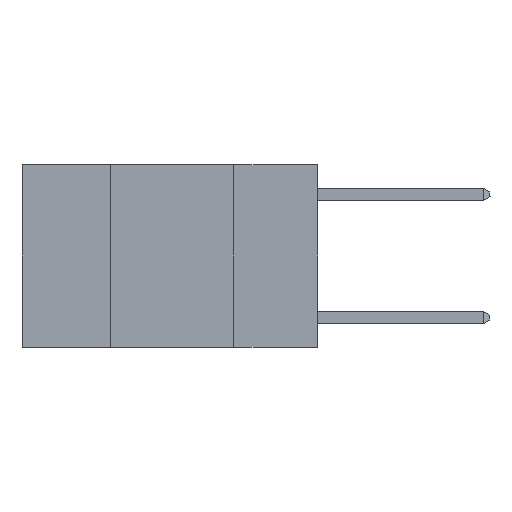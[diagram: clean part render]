
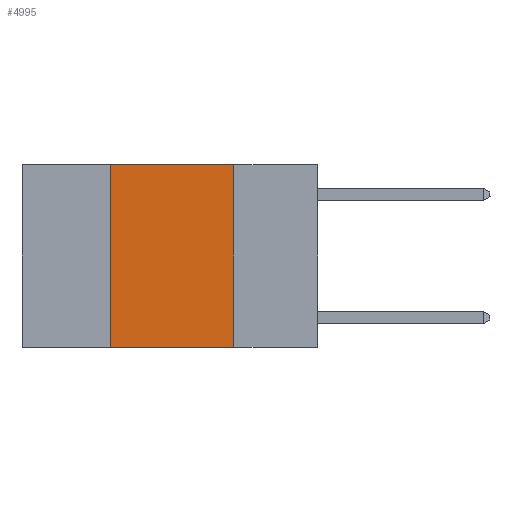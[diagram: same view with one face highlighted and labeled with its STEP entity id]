
A CAD part, left-side view. The second image highlights one B-rep face of the part: STEP entity #4995.
In plain terms, the highlighted planar face has unit normal (-1, 0, 0).
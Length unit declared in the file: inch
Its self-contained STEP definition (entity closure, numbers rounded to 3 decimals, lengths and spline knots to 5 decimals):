
#2 = VECTOR ( 'NONE', #11920, 39.37008 ) ;
#443 = EDGE_CURVE ( 'NONE', #1747, #7035, #8086, .T. ) ;
#449 = VECTOR ( 'NONE', #13434, 39.37008 ) ;
#651 = CARTESIAN_POINT ( 'NONE',  ( 0., 0.42, 0. ) ) ;
#919 = EDGE_LOOP ( 'NONE', ( #1502, #14373, #14010, #5886 ) ) ;
#1212 = VERTEX_POINT ( 'NONE', #9238 ) ;
#1342 = EDGE_CURVE ( 'NONE', #14211, #1212, #10593, .T. ) ;
#1502 = ORIENTED_EDGE ( 'NONE', *, *, #1342, .F. ) ;
#1544 = CARTESIAN_POINT ( 'NONE',  ( 0., 0.17, 0. ) ) ;
#1636 = VECTOR ( 'NONE', #14816, 39.37008 ) ;
#1741 = VECTOR ( 'NONE', #5179, 39.37008 ) ;
#1747 = VERTEX_POINT ( 'NONE', #7287 ) ;
#1995 = CARTESIAN_POINT ( 'NONE',  ( 0., 0.6, 0. ) ) ;
#2073 = LINE ( 'NONE', #7493, #1636 ) ;
#3516 = LINE ( 'NONE', #5611, #2 ) ;
#4530 = DIRECTION ( 'NONE',  ( 0., 0., -1. ) ) ;
#4995 = ADVANCED_FACE ( 'NONE', ( #9917 ), #9570, .F. ) ;
#5179 = DIRECTION ( 'NONE',  ( 0., 0., 1. ) ) ;
#5611 = CARTESIAN_POINT ( 'NONE',  ( 0., 0.6, 0. ) ) ;
#5886 = ORIENTED_EDGE ( 'NONE', *, *, #12332, .T. ) ;
#6142 = EDGE_CURVE ( 'NONE', #7035, #14211, #3516, .T. ) ;
#7035 = VERTEX_POINT ( 'NONE', #651 ) ;
#7287 = CARTESIAN_POINT ( 'NONE',  ( 0., 0.42, -0.37 ) ) ;
#7493 = CARTESIAN_POINT ( 'NONE',  ( 0., 0.6, -0.37 ) ) ;
#8086 = LINE ( 'NONE', #10122, #1741 ) ;
#9238 = CARTESIAN_POINT ( 'NONE',  ( 0., 0.17, -0.37 ) ) ;
#9570 = PLANE ( 'NONE',  #9814 ) ;
#9814 = AXIS2_PLACEMENT_3D ( 'NONE', #1995, #12058, #4530 ) ;
#9917 = FACE_OUTER_BOUND ( 'NONE', #919, .T. ) ;
#10122 = CARTESIAN_POINT ( 'NONE',  ( 0., 0.42, 0. ) ) ;
#10593 = LINE ( 'NONE', #1544, #449 ) ;
#11920 = DIRECTION ( 'NONE',  ( 0., -1., 0. ) ) ;
#12058 = DIRECTION ( 'NONE',  ( 1., 0., 0. ) ) ;
#12332 = EDGE_CURVE ( 'NONE', #1747, #1212, #2073, .T. ) ;
#13434 = DIRECTION ( 'NONE',  ( 0., 0., -1. ) ) ;
#14010 = ORIENTED_EDGE ( 'NONE', *, *, #443, .F. ) ;
#14211 = VERTEX_POINT ( 'NONE', #15823 ) ;
#14373 = ORIENTED_EDGE ( 'NONE', *, *, #6142, .F. ) ;
#14816 = DIRECTION ( 'NONE',  ( 0., -1., 0. ) ) ;
#15823 = CARTESIAN_POINT ( 'NONE',  ( 0., 0.17, 0. ) ) ;
